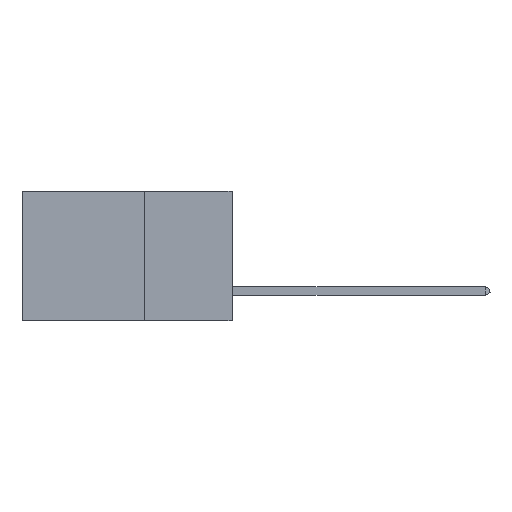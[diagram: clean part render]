
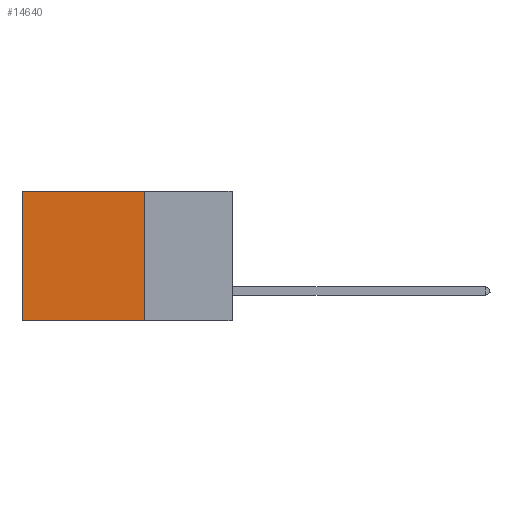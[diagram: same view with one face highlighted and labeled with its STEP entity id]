
A CAD part, left-side view. The second image highlights one B-rep face of the part: STEP entity #14640.
In plain terms, the highlighted planar face has unit normal (-1, 0, 0).
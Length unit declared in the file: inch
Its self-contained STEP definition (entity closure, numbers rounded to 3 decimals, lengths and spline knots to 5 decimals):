
#775 = LINE ( 'NONE', #24364, #26517 ) ;
#1721 = DIRECTION ( 'NONE',  ( 0., 1., 0. ) ) ;
#2257 = CARTESIAN_POINT ( 'NONE',  ( 0.2875, 0.6, 0. ) ) ;
#2457 = CARTESIAN_POINT ( 'NONE',  ( 0.2875, 0.6, 0. ) ) ;
#3359 = CARTESIAN_POINT ( 'NONE',  ( 0.2875, 0.25, -0.37 ) ) ;
#3736 = VECTOR ( 'NONE', #18915, 39.37008 ) ;
#3835 = EDGE_CURVE ( 'NONE', #20978, #16588, #19415, .T. ) ;
#6163 = ORIENTED_EDGE ( 'NONE', *, *, #24219, .F. ) ;
#6520 = CARTESIAN_POINT ( 'NONE',  ( 0.2875, 0.25, -0.37 ) ) ;
#6760 = ORIENTED_EDGE ( 'NONE', *, *, #14413, .T. ) ;
#6913 = PLANE ( 'NONE',  #24502 ) ;
#8420 = DIRECTION ( 'NONE',  ( 0., 0., -1. ) ) ;
#8502 = VECTOR ( 'NONE', #8420, 39.37008 ) ;
#8510 = ORIENTED_EDGE ( 'NONE', *, *, #3835, .F. ) ;
#8674 = ORIENTED_EDGE ( 'NONE', *, *, #21010, .T. ) ;
#8776 = CARTESIAN_POINT ( 'NONE',  ( 0.2875, 0.6, -0.37 ) ) ;
#8840 = FACE_OUTER_BOUND ( 'NONE', #15386, .T. ) ;
#9021 = VECTOR ( 'NONE', #12556, 39.37008 ) ;
#10130 = LINE ( 'NONE', #2457, #3736 ) ;
#12556 = DIRECTION ( 'NONE',  ( 0., 1., 0. ) ) ;
#14248 = CARTESIAN_POINT ( 'NONE',  ( 0.2875, 0.25, 0. ) ) ;
#14413 = EDGE_CURVE ( 'NONE', #20978, #18141, #775, .T. ) ;
#14640 = ADVANCED_FACE ( 'NONE', ( #8840 ), #6913, .F. ) ;
#14678 = VERTEX_POINT ( 'NONE', #8776 ) ;
#14799 = CARTESIAN_POINT ( 'NONE',  ( 0.2875, 0.25, 0. ) ) ;
#15115 = LINE ( 'NONE', #3359, #9021 ) ;
#15321 = DIRECTION ( 'NONE',  ( 0., 0., -1. ) ) ;
#15386 = EDGE_LOOP ( 'NONE', ( #8674, #6163, #8510, #6760 ) ) ;
#16588 = VERTEX_POINT ( 'NONE', #6520 ) ;
#18141 = VERTEX_POINT ( 'NONE', #2257 ) ;
#18915 = DIRECTION ( 'NONE',  ( 0., 0., -1. ) ) ;
#19415 = LINE ( 'NONE', #14248, #8502 ) ;
#20978 = VERTEX_POINT ( 'NONE', #14799 ) ;
#21010 = EDGE_CURVE ( 'NONE', #18141, #14678, #10130, .T. ) ;
#21179 = CARTESIAN_POINT ( 'NONE',  ( 0.2875, 0.25, 0. ) ) ;
#24219 = EDGE_CURVE ( 'NONE', #16588, #14678, #15115, .T. ) ;
#24364 = CARTESIAN_POINT ( 'NONE',  ( 0.2875, 0.25, 0. ) ) ;
#24502 = AXIS2_PLACEMENT_3D ( 'NONE', #21179, #25337, #15321 ) ;
#25337 = DIRECTION ( 'NONE',  ( 1., 0., 0. ) ) ;
#26517 = VECTOR ( 'NONE', #1721, 39.37008 ) ;
